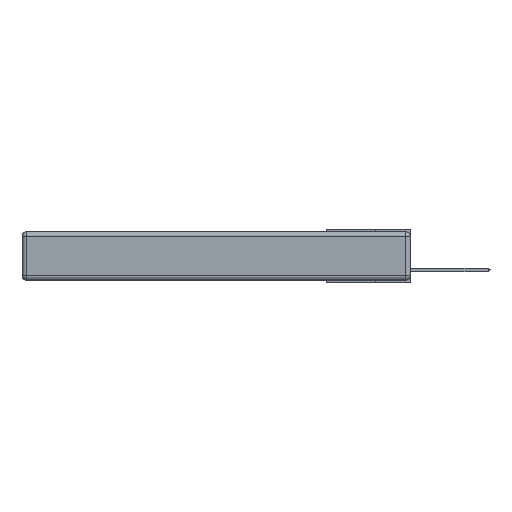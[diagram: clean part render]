
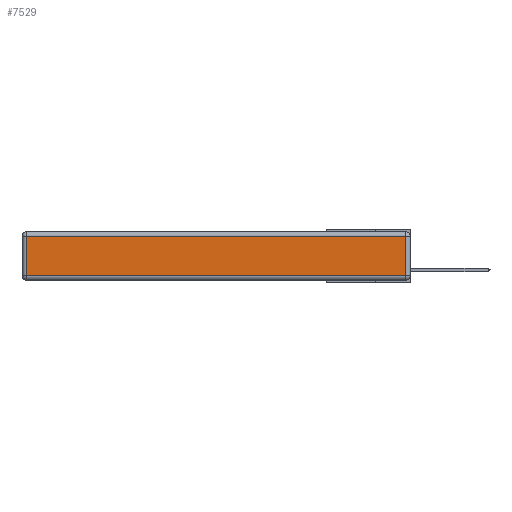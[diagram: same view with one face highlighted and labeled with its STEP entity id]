
A CAD part, left-side view. The second image highlights one B-rep face of the part: STEP entity #7529.
In plain terms, the highlighted planar face has unit normal (-1, 0, 0).
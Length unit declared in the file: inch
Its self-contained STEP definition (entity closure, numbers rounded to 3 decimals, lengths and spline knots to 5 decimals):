
#1154 = EDGE_CURVE ( 'NONE', #20843, #6169, #7925, .T. ) ;
#4067 = VECTOR ( 'NONE', #5253, 39.37008 ) ;
#4437 = CARTESIAN_POINT ( 'NONE',  ( 0., 2.72, -0.343 ) ) ;
#5096 = EDGE_LOOP ( 'NONE', ( #9583, #23189, #28033, #5409 ) ) ;
#5253 = DIRECTION ( 'NONE',  ( 0., 0., 1. ) ) ;
#5409 = ORIENTED_EDGE ( 'NONE', *, *, #1154, .T. ) ;
#5414 = FACE_OUTER_BOUND ( 'NONE', #5096, .T. ) ;
#6169 = VERTEX_POINT ( 'NONE', #16825 ) ;
#6983 = CARTESIAN_POINT ( 'NONE',  ( 0., 0., -0.343 ) ) ;
#7039 = VERTEX_POINT ( 'NONE', #19642 ) ;
#7169 = VECTOR ( 'NONE', #16990, 39.37008 ) ;
#7529 = ADVANCED_FACE ( 'NONE', ( #5414 ), #26768, .T. ) ;
#7925 = LINE ( 'NONE', #4437, #26095 ) ;
#9583 = ORIENTED_EDGE ( 'NONE', *, *, #9734, .T. ) ;
#9734 = EDGE_CURVE ( 'NONE', #6169, #7039, #22524, .T. ) ;
#10788 = CARTESIAN_POINT ( 'NONE',  ( 0., 2.72, -0.03 ) ) ;
#10886 = VECTOR ( 'NONE', #16942, 39.37008 ) ;
#12444 = AXIS2_PLACEMENT_3D ( 'NONE', #6983, #20321, #24844 ) ;
#14091 = EDGE_CURVE ( 'NONE', #24288, #20843, #17829, .T. ) ;
#14405 = LINE ( 'NONE', #18392, #4067 ) ;
#14579 = EDGE_CURVE ( 'NONE', #7039, #24288, #14405, .T. ) ;
#15584 = DIRECTION ( 'NONE',  ( 0., 0., -1. ) ) ;
#16825 = CARTESIAN_POINT ( 'NONE',  ( 0., 2.72, -0.313 ) ) ;
#16942 = DIRECTION ( 'NONE',  ( 0., -1., 0. ) ) ;
#16990 = DIRECTION ( 'NONE',  ( 0., 1., 0. ) ) ;
#17829 = LINE ( 'NONE', #19173, #7169 ) ;
#18392 = CARTESIAN_POINT ( 'NONE',  ( 0., 0.03, -0.343 ) ) ;
#19173 = CARTESIAN_POINT ( 'NONE',  ( 0., 2.75, -0.03 ) ) ;
#19642 = CARTESIAN_POINT ( 'NONE',  ( 0., 0.03, -0.313 ) ) ;
#20321 = DIRECTION ( 'NONE',  ( -1., 0., 0. ) ) ;
#20843 = VERTEX_POINT ( 'NONE', #10788 ) ;
#22524 = LINE ( 'NONE', #23435, #10886 ) ;
#23189 = ORIENTED_EDGE ( 'NONE', *, *, #14579, .T. ) ;
#23435 = CARTESIAN_POINT ( 'NONE',  ( 0., 0., -0.313 ) ) ;
#24288 = VERTEX_POINT ( 'NONE', #25413 ) ;
#24844 = DIRECTION ( 'NONE',  ( 0., 0., 1. ) ) ;
#25413 = CARTESIAN_POINT ( 'NONE',  ( 0., 0.03, -0.03 ) ) ;
#26095 = VECTOR ( 'NONE', #15584, 39.37008 ) ;
#26768 = PLANE ( 'NONE',  #12444 ) ;
#28033 = ORIENTED_EDGE ( 'NONE', *, *, #14091, .T. ) ;
